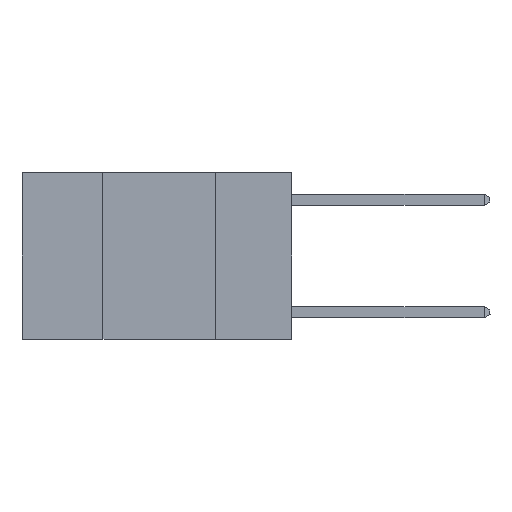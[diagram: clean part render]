
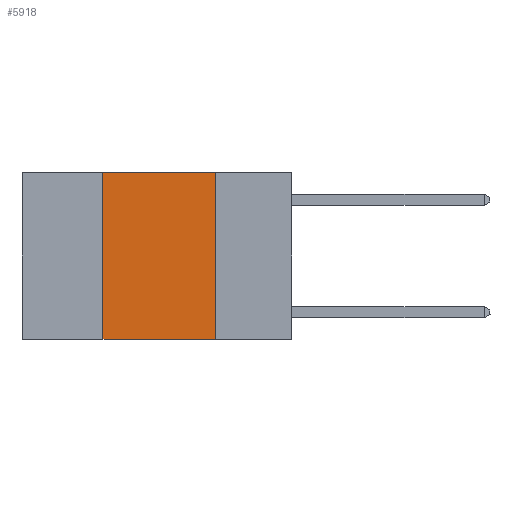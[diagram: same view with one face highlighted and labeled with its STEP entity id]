
A CAD part, left-side view. The second image highlights one B-rep face of the part: STEP entity #5918.
In plain terms, the highlighted planar face has unit normal (-1, 0, 0).
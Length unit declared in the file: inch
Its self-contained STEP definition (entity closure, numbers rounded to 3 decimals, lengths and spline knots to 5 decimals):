
#81 = EDGE_CURVE ( 'NONE', #5316, #10023, #13159, .T. ) ;
#693 = EDGE_LOOP ( 'NONE', ( #20610, #1606, #25074, #2913 ) ) ;
#1044 = VECTOR ( 'NONE', #12206, 39.37008 ) ;
#1606 = ORIENTED_EDGE ( 'NONE', *, *, #81, .F. ) ;
#2896 = LINE ( 'NONE', #11339, #7904 ) ;
#2913 = ORIENTED_EDGE ( 'NONE', *, *, #7260, .T. ) ;
#3227 = CARTESIAN_POINT ( 'NONE',  ( 0., 0.17, 0. ) ) ;
#3518 = CARTESIAN_POINT ( 'NONE',  ( 0., 0.6, 0. ) ) ;
#5316 = VERTEX_POINT ( 'NONE', #10862 ) ;
#5622 = DIRECTION ( 'NONE',  ( 0., -1., 0. ) ) ;
#5918 = ADVANCED_FACE ( 'NONE', ( #18405 ), #19234, .F. ) ;
#5940 = CARTESIAN_POINT ( 'NONE',  ( 0., 0.17, -0.37 ) ) ;
#6674 = DIRECTION ( 'NONE',  ( 1., 0., 0. ) ) ;
#7186 = DIRECTION ( 'NONE',  ( 0., 0., -1. ) ) ;
#7260 = EDGE_CURVE ( 'NONE', #25946, #16749, #9146, .T. ) ;
#7904 = VECTOR ( 'NONE', #7186, 39.37008 ) ;
#8572 = CARTESIAN_POINT ( 'NONE',  ( 0., 0.6, -0.37 ) ) ;
#9146 = LINE ( 'NONE', #8572, #14082 ) ;
#10023 = VERTEX_POINT ( 'NONE', #3227 ) ;
#10837 = CARTESIAN_POINT ( 'NONE',  ( 0., 0.6, 0. ) ) ;
#10862 = CARTESIAN_POINT ( 'NONE',  ( 0., 0.42, 0. ) ) ;
#11339 = CARTESIAN_POINT ( 'NONE',  ( 0., 0.17, 0. ) ) ;
#11750 = LINE ( 'NONE', #22534, #1044 ) ;
#12002 = CARTESIAN_POINT ( 'NONE',  ( 0., 0.42, -0.37 ) ) ;
#12206 = DIRECTION ( 'NONE',  ( 0., 0., 1. ) ) ;
#13159 = LINE ( 'NONE', #3518, #23514 ) ;
#14082 = VECTOR ( 'NONE', #25140, 39.37008 ) ;
#16423 = EDGE_CURVE ( 'NONE', #10023, #16749, #2896, .T. ) ;
#16749 = VERTEX_POINT ( 'NONE', #5940 ) ;
#18405 = FACE_OUTER_BOUND ( 'NONE', #693, .T. ) ;
#19234 = PLANE ( 'NONE',  #25663 ) ;
#19682 = EDGE_CURVE ( 'NONE', #25946, #5316, #11750, .T. ) ;
#20610 = ORIENTED_EDGE ( 'NONE', *, *, #16423, .F. ) ;
#21321 = DIRECTION ( 'NONE',  ( 0., 0., -1. ) ) ;
#22534 = CARTESIAN_POINT ( 'NONE',  ( 0., 0.42, 0. ) ) ;
#23514 = VECTOR ( 'NONE', #5622, 39.37008 ) ;
#25074 = ORIENTED_EDGE ( 'NONE', *, *, #19682, .F. ) ;
#25140 = DIRECTION ( 'NONE',  ( 0., -1., 0. ) ) ;
#25663 = AXIS2_PLACEMENT_3D ( 'NONE', #10837, #6674, #21321 ) ;
#25946 = VERTEX_POINT ( 'NONE', #12002 ) ;
